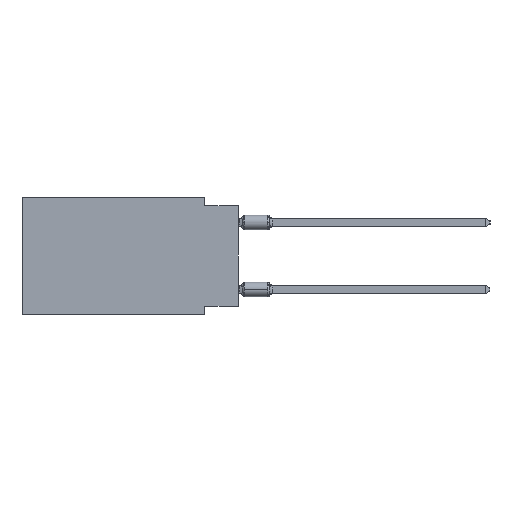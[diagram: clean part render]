
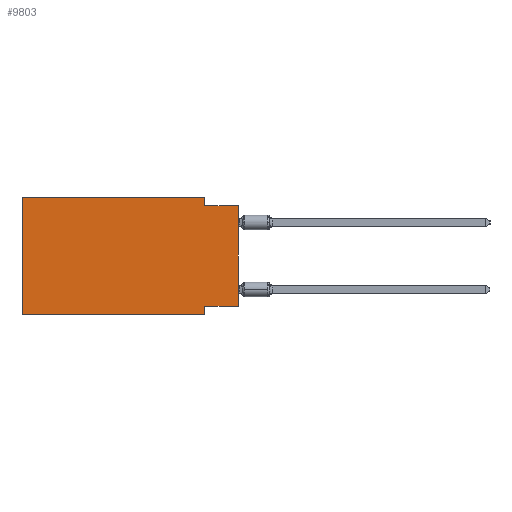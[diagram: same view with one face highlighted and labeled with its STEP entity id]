
A CAD part, left-side view. The second image highlights one B-rep face of the part: STEP entity #9803.
In plain terms, the highlighted planar face has unit normal (-1, 0, 0).
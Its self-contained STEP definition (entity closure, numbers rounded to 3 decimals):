
#218 = EDGE_CURVE ( 'NONE', #6912, #2228, #6524, .T. ) ;
#448 = LINE ( 'NONE', #15548, #7322 ) ;
#674 = DIRECTION ( 'NONE',  ( 0., -1., 0. ) ) ;
#1184 = AXIS2_PLACEMENT_3D ( 'NONE', #6115, #8639, #3589 ) ;
#1390 = EDGE_LOOP ( 'NONE', ( #3743, #15339, #10813, #11248, #10726, #11758, #2896, #9690 ) ) ;
#1424 = VECTOR ( 'NONE', #7603, 1000. ) ;
#1804 = VECTOR ( 'NONE', #6826, 1000. ) ;
#1904 = CARTESIAN_POINT ( 'NONE',  ( 0., 16.383, 0. ) ) ;
#2020 = VECTOR ( 'NONE', #674, 1000. ) ;
#2100 = FACE_OUTER_BOUND ( 'NONE', #1390, .T. ) ;
#2228 = VERTEX_POINT ( 'NONE', #13897 ) ;
#2420 = LINE ( 'NONE', #14110, #9310 ) ;
#2849 = CARTESIAN_POINT ( 'NONE',  ( 0., 0., -8.255 ) ) ;
#2896 = ORIENTED_EDGE ( 'NONE', *, *, #15474, .F. ) ;
#3017 = LINE ( 'NONE', #6798, #8742 ) ;
#3068 = EDGE_CURVE ( 'NONE', #2228, #4331, #2420, .T. ) ;
#3510 = EDGE_CURVE ( 'NONE', #9658, #6752, #9355, .T. ) ;
#3589 = DIRECTION ( 'NONE',  ( 0., 0., -1. ) ) ;
#3743 = ORIENTED_EDGE ( 'NONE', *, *, #3510, .T. ) ;
#4004 = EDGE_CURVE ( 'NONE', #9658, #12826, #448, .T. ) ;
#4331 = VERTEX_POINT ( 'NONE', #10222 ) ;
#4340 = VECTOR ( 'NONE', #14014, 1000. ) ;
#5553 = DIRECTION ( 'NONE',  ( 0., 1., 0. ) ) ;
#5937 = CARTESIAN_POINT ( 'NONE',  ( 0., 16.383, -8.89 ) ) ;
#6115 = CARTESIAN_POINT ( 'NONE',  ( 0., 16.383, 0. ) ) ;
#6524 = LINE ( 'NONE', #8804, #4340 ) ;
#6635 = CARTESIAN_POINT ( 'NONE',  ( 0., 16.383, 0. ) ) ;
#6673 = VERTEX_POINT ( 'NONE', #8411 ) ;
#6752 = VERTEX_POINT ( 'NONE', #15212 ) ;
#6798 = CARTESIAN_POINT ( 'NONE',  ( 0., 2.54, -8.89 ) ) ;
#6826 = DIRECTION ( 'NONE',  ( 0., 0., 1. ) ) ;
#6912 = VERTEX_POINT ( 'NONE', #6635 ) ;
#7322 = VECTOR ( 'NONE', #5553, 1000. ) ;
#7603 = DIRECTION ( 'NONE',  ( 0., -1., 0. ) ) ;
#8085 = CARTESIAN_POINT ( 'NONE',  ( 0., 0., 0. ) ) ;
#8128 = VECTOR ( 'NONE', #14927, 1000. ) ;
#8411 = CARTESIAN_POINT ( 'NONE',  ( 0., 2.54, -8.89 ) ) ;
#8612 = CARTESIAN_POINT ( 'NONE',  ( 0., 0., -0.635 ) ) ;
#8633 = EDGE_CURVE ( 'NONE', #16530, #6673, #14943, .T. ) ;
#8639 = DIRECTION ( 'NONE',  ( 1., 0., 0. ) ) ;
#8742 = VECTOR ( 'NONE', #13358, 1000. ) ;
#8804 = CARTESIAN_POINT ( 'NONE',  ( 0., 16.383, 0. ) ) ;
#8888 = DIRECTION ( 'NONE',  ( 0., 0., -1. ) ) ;
#9310 = VECTOR ( 'NONE', #8888, 1000. ) ;
#9355 = LINE ( 'NONE', #8085, #1804 ) ;
#9658 = VERTEX_POINT ( 'NONE', #2849 ) ;
#9690 = ORIENTED_EDGE ( 'NONE', *, *, #4004, .F. ) ;
#9803 = ADVANCED_FACE ( 'NONE', ( #2100 ), #11085, .F. ) ;
#10100 = CARTESIAN_POINT ( 'NONE',  ( 0., 2.54, -8.255 ) ) ;
#10170 = EDGE_CURVE ( 'NONE', #16530, #6912, #13496, .T. ) ;
#10222 = CARTESIAN_POINT ( 'NONE',  ( 0., 2.54, -0.635 ) ) ;
#10280 = EDGE_CURVE ( 'NONE', #4331, #6752, #16585, .T. ) ;
#10726 = ORIENTED_EDGE ( 'NONE', *, *, #10170, .F. ) ;
#10813 = ORIENTED_EDGE ( 'NONE', *, *, #3068, .F. ) ;
#11085 = PLANE ( 'NONE',  #1184 ) ;
#11248 = ORIENTED_EDGE ( 'NONE', *, *, #218, .F. ) ;
#11758 = ORIENTED_EDGE ( 'NONE', *, *, #8633, .T. ) ;
#12826 = VERTEX_POINT ( 'NONE', #10100 ) ;
#13358 = DIRECTION ( 'NONE',  ( 0., 0., -1. ) ) ;
#13496 = LINE ( 'NONE', #1904, #8128 ) ;
#13897 = CARTESIAN_POINT ( 'NONE',  ( 0., 2.54, 0. ) ) ;
#14014 = DIRECTION ( 'NONE',  ( 0., -1., 0. ) ) ;
#14110 = CARTESIAN_POINT ( 'NONE',  ( 0., 2.54, 0. ) ) ;
#14351 = CARTESIAN_POINT ( 'NONE',  ( 0., 16.383, -8.89 ) ) ;
#14927 = DIRECTION ( 'NONE',  ( 0., 0., 1. ) ) ;
#14943 = LINE ( 'NONE', #5937, #2020 ) ;
#15212 = CARTESIAN_POINT ( 'NONE',  ( 0., 0., -0.635 ) ) ;
#15339 = ORIENTED_EDGE ( 'NONE', *, *, #10280, .F. ) ;
#15474 = EDGE_CURVE ( 'NONE', #12826, #6673, #3017, .T. ) ;
#15548 = CARTESIAN_POINT ( 'NONE',  ( 0., 0., -8.255 ) ) ;
#16530 = VERTEX_POINT ( 'NONE', #14351 ) ;
#16585 = LINE ( 'NONE', #8612, #1424 ) ;
